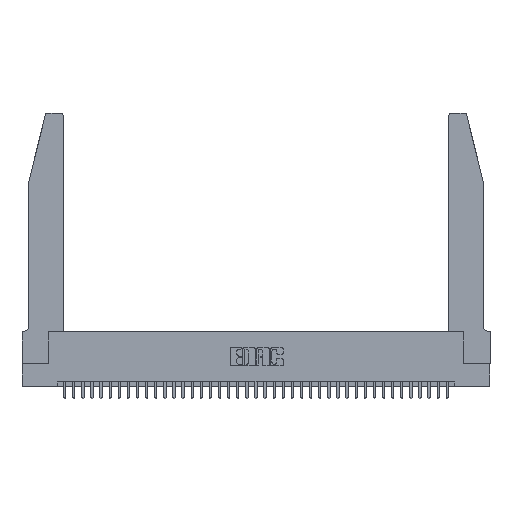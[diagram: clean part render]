
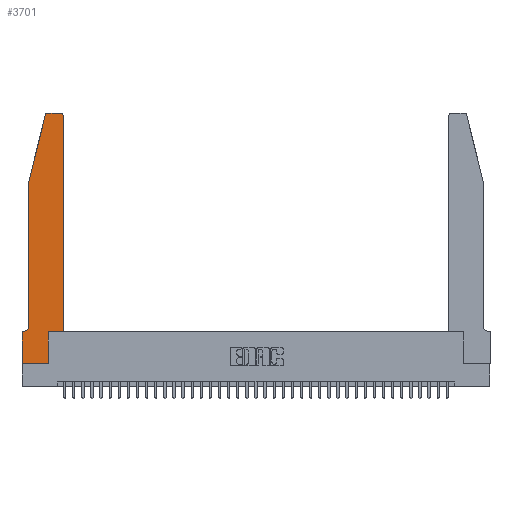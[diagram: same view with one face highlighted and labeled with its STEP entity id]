
A CAD part, top view. The second image highlights one B-rep face of the part: STEP entity #3701.
In plain terms, the highlighted planar face has unit normal (0, 0, 1).
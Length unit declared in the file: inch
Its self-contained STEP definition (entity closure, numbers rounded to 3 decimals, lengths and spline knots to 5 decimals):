
#794 = EDGE_CURVE ( 'NONE', #25652, #25342, #25755, .T. ) ;
#1041 = DIRECTION ( 'NONE',  ( 1., 0., 0. ) ) ;
#1202 = ORIENTED_EDGE ( 'NONE', *, *, #34939, .T. ) ;
#2660 = ORIENTED_EDGE ( 'NONE', *, *, #11709, .T. ) ;
#3054 = CARTESIAN_POINT ( 'NONE',  ( 0.0755, 2., 0.37 ) ) ;
#3701 = ADVANCED_FACE ( 'NONE', ( #31476 ), #36555, .T. ) ;
#5142 = CARTESIAN_POINT ( 'NONE',  ( 0.4505, 0.35, 0.37 ) ) ;
#5250 = ORIENTED_EDGE ( 'NONE', *, *, #29625, .T. ) ;
#5386 = EDGE_CURVE ( 'NONE', #19175, #37126, #13885, .T. ) ;
#5935 = DIRECTION ( 'NONE',  ( -0.239, -0.971, 0. ) ) ;
#6050 = LINE ( 'NONE', #14409, #20080 ) ;
#6173 = VERTEX_POINT ( 'NONE', #15101 ) ;
#6363 = VECTOR ( 'NONE', #16667, 39.37008 ) ;
#6626 = DIRECTION ( 'NONE',  ( 0., 0., -1. ) ) ;
#7388 = CARTESIAN_POINT ( 'NONE',  ( 0.4205, 2.72, 0.37 ) ) ;
#7848 = EDGE_LOOP ( 'NONE', ( #1202, #2660, #23015, #28528, #34599, #37508, #9718, #9901, #37915, #22116, #10364, #5250 ) ) ;
#8500 = CARTESIAN_POINT ( 'NONE',  ( 0.4205, 2.75, 0.37 ) ) ;
#9718 = ORIENTED_EDGE ( 'NONE', *, *, #29386, .T. ) ;
#9901 = ORIENTED_EDGE ( 'NONE', *, *, #20959, .T. ) ;
#10108 = DIRECTION ( 'NONE',  ( 0., 1., 0. ) ) ;
#10290 = CARTESIAN_POINT ( 'NONE',  ( 0.284, 2.72, 0.37 ) ) ;
#10364 = ORIENTED_EDGE ( 'NONE', *, *, #37691, .T. ) ;
#10418 = DIRECTION ( 'NONE',  ( 1., 0., 0. ) ) ;
#11108 = DIRECTION ( 'NONE',  ( 1., 0., 0. ) ) ;
#11709 = EDGE_CURVE ( 'NONE', #26316, #36976, #17944, .T. ) ;
#12607 = VERTEX_POINT ( 'NONE', #32557 ) ;
#12693 = CARTESIAN_POINT ( 'NONE',  ( 0.0055, 0.35, 0.37 ) ) ;
#12958 = VECTOR ( 'NONE', #27779, 39.37008 ) ;
#13331 = DIRECTION ( 'NONE',  ( 1., 0., 0. ) ) ;
#13559 = CARTESIAN_POINT ( 'NONE',  ( 0., 0., 0.37 ) ) ;
#13885 = LINE ( 'NONE', #24827, #12958 ) ;
#14409 = CARTESIAN_POINT ( 'NONE',  ( 0.2605, 2.75, 0.37 ) ) ;
#15101 = CARTESIAN_POINT ( 'NONE',  ( 0.4505, 2.72, 0.37 ) ) ;
#15146 = LINE ( 'NONE', #26755, #22091 ) ;
#15612 = VECTOR ( 'NONE', #10108, 39.37008 ) ;
#15970 = VERTEX_POINT ( 'NONE', #13559 ) ;
#16072 = CARTESIAN_POINT ( 'NONE',  ( 0.0755, 0.42, 0.37 ) ) ;
#16667 = DIRECTION ( 'NONE',  ( 0., 1., 0. ) ) ;
#16996 = CARTESIAN_POINT ( 'NONE',  ( 0., 0., 0.37 ) ) ;
#17454 = EDGE_CURVE ( 'NONE', #12607, #19175, #24394, .T. ) ;
#17869 = VECTOR ( 'NONE', #28701, 39.37008 ) ;
#17944 = CIRCLE ( 'NONE', #33481, 0.03 ) ;
#18035 = VERTEX_POINT ( 'NONE', #21533 ) ;
#18985 = DIRECTION ( 'NONE',  ( 0., 0., 1. ) ) ;
#19175 = VERTEX_POINT ( 'NONE', #24157 ) ;
#19272 = CIRCLE ( 'NONE', #20055, 0.03 ) ;
#19758 = VECTOR ( 'NONE', #21116, 39.37008 ) ;
#20055 = AXIS2_PLACEMENT_3D ( 'NONE', #7388, #28167, #10418 ) ;
#20080 = VECTOR ( 'NONE', #32018, 39.37008 ) ;
#20959 = EDGE_CURVE ( 'NONE', #15970, #12607, #37201, .T. ) ;
#21116 = DIRECTION ( 'NONE',  ( 0., -1., 0. ) ) ;
#21195 = EDGE_CURVE ( 'NONE', #36976, #18035, #15146, .T. ) ;
#21533 = CARTESIAN_POINT ( 'NONE',  ( 0.0755, 2., 0.37 ) ) ;
#21644 = VECTOR ( 'NONE', #11108, 39.37008 ) ;
#21909 = VECTOR ( 'NONE', #23926, 39.37008 ) ;
#22091 = VECTOR ( 'NONE', #5935, 39.37008 ) ;
#22116 = ORIENTED_EDGE ( 'NONE', *, *, #5386, .T. ) ;
#22248 = LINE ( 'NONE', #34227, #6363 ) ;
#22259 = CARTESIAN_POINT ( 'NONE',  ( 0.25487, 2.72718, 0.37 ) ) ;
#22315 = VERTEX_POINT ( 'NONE', #8500 ) ;
#22780 = CARTESIAN_POINT ( 'NONE',  ( 0.0755, 0.35, 0.37 ) ) ;
#23015 = ORIENTED_EDGE ( 'NONE', *, *, #21195, .T. ) ;
#23503 = AXIS2_PLACEMENT_3D ( 'NONE', #27772, #18985, #1041 ) ;
#23661 = EDGE_CURVE ( 'NONE', #36949, #25652, #37436, .T. ) ;
#23926 = DIRECTION ( 'NONE',  ( 0., -1., 0. ) ) ;
#24068 = CARTESIAN_POINT ( 'NONE',  ( 0., 0., 0.37 ) ) ;
#24157 = CARTESIAN_POINT ( 'NONE',  ( 0.2865, 0.35, 0.37 ) ) ;
#24394 = LINE ( 'NONE', #30820, #15612 ) ;
#24466 = CARTESIAN_POINT ( 'NONE',  ( 0.0055, 0.42, 0.37 ) ) ;
#24646 = AXIS2_PLACEMENT_3D ( 'NONE', #24466, #6626, #27428 ) ;
#24827 = CARTESIAN_POINT ( 'NONE',  ( 0.4505, 0.35, 0.37 ) ) ;
#25342 = VERTEX_POINT ( 'NONE', #37892 ) ;
#25652 = VERTEX_POINT ( 'NONE', #12693 ) ;
#25755 = LINE ( 'NONE', #22780, #17869 ) ;
#26316 = VERTEX_POINT ( 'NONE', #36796 ) ;
#26755 = CARTESIAN_POINT ( 'NONE',  ( 0.0755, 2., 0.37 ) ) ;
#27428 = DIRECTION ( 'NONE',  ( -1., 0., 0. ) ) ;
#27772 = CARTESIAN_POINT ( 'NONE',  ( 0., 0.35, 0.37 ) ) ;
#27779 = DIRECTION ( 'NONE',  ( 1., 0., 0. ) ) ;
#28167 = DIRECTION ( 'NONE',  ( 0., 0., 1. ) ) ;
#28528 = ORIENTED_EDGE ( 'NONE', *, *, #31334, .T. ) ;
#28701 = DIRECTION ( 'NONE',  ( -1., 0., 0. ) ) ;
#29386 = EDGE_CURVE ( 'NONE', #25342, #15970, #35330, .T. ) ;
#29625 = EDGE_CURVE ( 'NONE', #6173, #22315, #19272, .T. ) ;
#29733 = LINE ( 'NONE', #3054, #21909 ) ;
#30820 = CARTESIAN_POINT ( 'NONE',  ( 0.2865, 0.35, 0.37 ) ) ;
#30987 = DIRECTION ( 'NONE',  ( 0., 0., 1. ) ) ;
#31334 = EDGE_CURVE ( 'NONE', #18035, #36949, #29733, .T. ) ;
#31476 = FACE_OUTER_BOUND ( 'NONE', #7848, .T. ) ;
#32018 = DIRECTION ( 'NONE',  ( -1., 0., 0. ) ) ;
#32557 = CARTESIAN_POINT ( 'NONE',  ( 0.2865, 0., 0.37 ) ) ;
#33481 = AXIS2_PLACEMENT_3D ( 'NONE', #10290, #30987, #13331 ) ;
#34227 = CARTESIAN_POINT ( 'NONE',  ( 0.4505, 0.35, 0.37 ) ) ;
#34599 = ORIENTED_EDGE ( 'NONE', *, *, #23661, .T. ) ;
#34939 = EDGE_CURVE ( 'NONE', #22315, #26316, #6050, .T. ) ;
#35330 = LINE ( 'NONE', #24068, #19758 ) ;
#36555 = PLANE ( 'NONE',  #23503 ) ;
#36796 = CARTESIAN_POINT ( 'NONE',  ( 0.284, 2.75, 0.37 ) ) ;
#36949 = VERTEX_POINT ( 'NONE', #16072 ) ;
#36976 = VERTEX_POINT ( 'NONE', #22259 ) ;
#37126 = VERTEX_POINT ( 'NONE', #5142 ) ;
#37201 = LINE ( 'NONE', #16996, #21644 ) ;
#37436 = CIRCLE ( 'NONE', #24646, 0.07 ) ;
#37508 = ORIENTED_EDGE ( 'NONE', *, *, #794, .T. ) ;
#37691 = EDGE_CURVE ( 'NONE', #37126, #6173, #22248, .T. ) ;
#37892 = CARTESIAN_POINT ( 'NONE',  ( 0., 0.35, 0.37 ) ) ;
#37915 = ORIENTED_EDGE ( 'NONE', *, *, #17454, .T. ) ;
